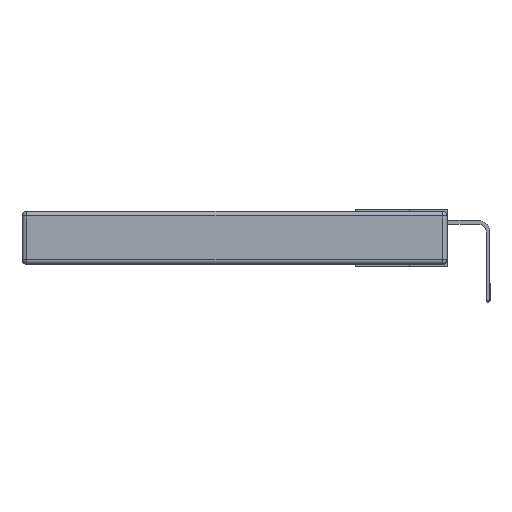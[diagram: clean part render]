
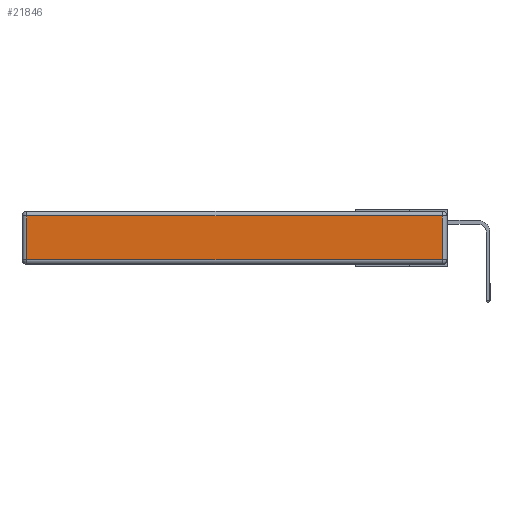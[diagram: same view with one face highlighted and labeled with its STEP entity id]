
A CAD part, left-side view. The second image highlights one B-rep face of the part: STEP entity #21846.
In plain terms, the highlighted planar face has unit normal (-1, 0, 0).
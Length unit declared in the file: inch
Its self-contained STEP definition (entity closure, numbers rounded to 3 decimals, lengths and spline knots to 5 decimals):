
#509 = VERTEX_POINT ( 'NONE', #9522 ) ;
#616 = LINE ( 'NONE', #27177, #24682 ) ;
#1591 = CARTESIAN_POINT ( 'NONE',  ( 0., 2.72, -0.343 ) ) ;
#2232 = CARTESIAN_POINT ( 'NONE',  ( 0., 0.03, -0.313 ) ) ;
#3139 = CARTESIAN_POINT ( 'NONE',  ( 0., 0., -0.343 ) ) ;
#3255 = CARTESIAN_POINT ( 'NONE',  ( 0., 2.72, -0.313 ) ) ;
#4557 = DIRECTION ( 'NONE',  ( 0., 0., 1. ) ) ;
#4571 = LINE ( 'NONE', #15361, #15147 ) ;
#5388 = ORIENTED_EDGE ( 'NONE', *, *, #13822, .T. ) ;
#5513 = DIRECTION ( 'NONE',  ( 0., 0., 1. ) ) ;
#6276 = ORIENTED_EDGE ( 'NONE', *, *, #12313, .T. ) ;
#7353 = LINE ( 'NONE', #12541, #7677 ) ;
#7517 = VERTEX_POINT ( 'NONE', #2232 ) ;
#7677 = VECTOR ( 'NONE', #8303, 39.37008 ) ;
#8303 = DIRECTION ( 'NONE',  ( 0., 1., 0. ) ) ;
#9522 = CARTESIAN_POINT ( 'NONE',  ( 0., 2.72, -0.03 ) ) ;
#9730 = DIRECTION ( 'NONE',  ( -1., 0., 0. ) ) ;
#10547 = ORIENTED_EDGE ( 'NONE', *, *, #14659, .T. ) ;
#12313 = EDGE_CURVE ( 'NONE', #509, #16096, #25415, .T. ) ;
#12541 = CARTESIAN_POINT ( 'NONE',  ( 0., 2.75, -0.03 ) ) ;
#13595 = VECTOR ( 'NONE', #14346, 39.37008 ) ;
#13641 = VERTEX_POINT ( 'NONE', #24784 ) ;
#13822 = EDGE_CURVE ( 'NONE', #16096, #7517, #616, .T. ) ;
#14346 = DIRECTION ( 'NONE',  ( 0., 0., -1. ) ) ;
#14659 = EDGE_CURVE ( 'NONE', #7517, #13641, #4571, .T. ) ;
#15147 = VECTOR ( 'NONE', #4557, 39.37008 ) ;
#15361 = CARTESIAN_POINT ( 'NONE',  ( 0., 0.03, -0.343 ) ) ;
#16096 = VERTEX_POINT ( 'NONE', #3255 ) ;
#17246 = ORIENTED_EDGE ( 'NONE', *, *, #25087, .T. ) ;
#19791 = AXIS2_PLACEMENT_3D ( 'NONE', #3139, #9730, #5513 ) ;
#20861 = EDGE_LOOP ( 'NONE', ( #5388, #10547, #17246, #6276 ) ) ;
#20921 = DIRECTION ( 'NONE',  ( 0., -1., 0. ) ) ;
#21846 = ADVANCED_FACE ( 'NONE', ( #24117 ), #26341, .T. ) ;
#24117 = FACE_OUTER_BOUND ( 'NONE', #20861, .T. ) ;
#24682 = VECTOR ( 'NONE', #20921, 39.37008 ) ;
#24784 = CARTESIAN_POINT ( 'NONE',  ( 0., 0.03, -0.03 ) ) ;
#25087 = EDGE_CURVE ( 'NONE', #13641, #509, #7353, .T. ) ;
#25415 = LINE ( 'NONE', #1591, #13595 ) ;
#26341 = PLANE ( 'NONE',  #19791 ) ;
#27177 = CARTESIAN_POINT ( 'NONE',  ( 0., 0., -0.313 ) ) ;
